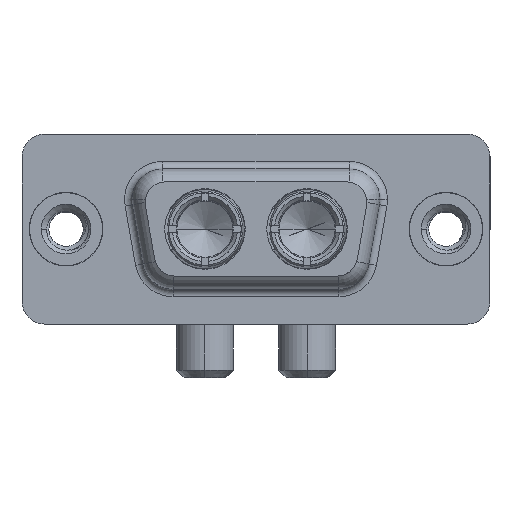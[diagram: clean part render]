
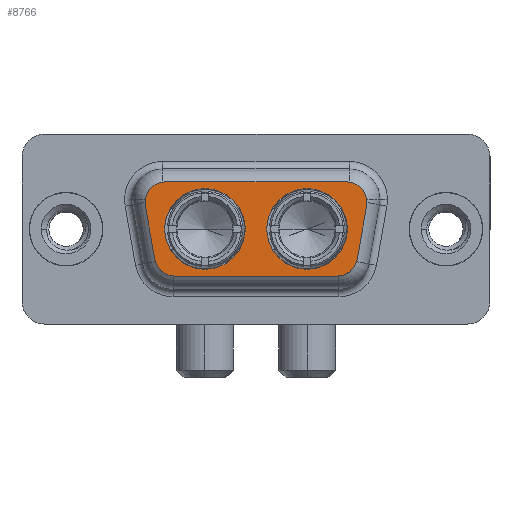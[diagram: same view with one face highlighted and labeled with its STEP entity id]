
A CAD part, top view. The second image highlights one B-rep face of the part: STEP entity #8766.
In plain terms, the highlighted planar face has unit normal (0, 0, 1).
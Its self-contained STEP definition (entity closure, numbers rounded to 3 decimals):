
#254 = DIRECTION ( 'NONE',  ( 0., 0., 1. ) ) ;
#322 = CARTESIAN_POINT ( 'NONE',  ( 9.14, 0., 6.2 ) ) ;
#446 = DIRECTION ( 'NONE',  ( 0., 0., 1. ) ) ;
#489 = VERTEX_POINT ( 'NONE', #9504 ) ;
#730 = CARTESIAN_POINT ( 'NONE',  ( 5.838, -1.984, 6.2 ) ) ;
#766 = CIRCLE ( 'NONE', #4537, 1.35 ) ;
#789 = VECTOR ( 'NONE', #3097, 1000. ) ;
#809 = CIRCLE ( 'NONE', #1787, 1.35 ) ;
#872 = ORIENTED_EDGE ( 'NONE', *, *, #11768, .T. ) ;
#908 = CARTESIAN_POINT ( 'NONE',  ( 7.167, -3.1, 6.2 ) ) ;
#1178 = EDGE_CURVE ( 'NONE', #6033, #6200, #5477, .T. ) ;
#1204 = VERTEX_POINT ( 'NONE', #908 ) ;
#1561 = DIRECTION ( 'NONE',  ( 0., 0., 1. ) ) ;
#1771 = VERTEX_POINT ( 'NONE', #10415 ) ;
#1781 = FACE_OUTER_BOUND ( 'NONE', #9798, .T. ) ;
#1787 = AXIS2_PLACEMENT_3D ( 'NONE', #3826, #3649, #8515 ) ;
#1828 = DIRECTION ( 'NONE',  ( 0., 0., 1. ) ) ;
#1871 = CARTESIAN_POINT ( 'NONE',  ( 18.45, 3.1, 6.2 ) ) ;
#1971 = AXIS2_PLACEMENT_3D ( 'NONE', #7436, #4839, #5643 ) ;
#2086 = DIRECTION ( 'NONE',  ( 0., 0., 1. ) ) ;
#2206 = DIRECTION ( 'NONE',  ( 1., 0., 0. ) ) ;
#2219 = LINE ( 'NONE', #11660, #789 ) ;
#2301 = ORIENTED_EDGE ( 'NONE', *, *, #11917, .T. ) ;
#2313 = ORIENTED_EDGE ( 'NONE', *, *, #7352, .T. ) ;
#2475 = EDGE_CURVE ( 'NONE', #4671, #489, #4843, .T. ) ;
#2494 = DIRECTION ( 'NONE',  ( 1., 0., 0. ) ) ;
#2518 = DIRECTION ( 'NONE',  ( 1., 0., 0. ) ) ;
#2545 = AXIS2_PLACEMENT_3D ( 'NONE', #7964, #2086, #4894 ) ;
#2638 = VERTEX_POINT ( 'NONE', #11983 ) ;
#2648 = AXIS2_PLACEMENT_3D ( 'NONE', #6838, #254, #4727 ) ;
#2899 = ORIENTED_EDGE ( 'NONE', *, *, #11365, .F. ) ;
#3053 = VERTEX_POINT ( 'NONE', #4282 ) ;
#3097 = DIRECTION ( 'NONE',  ( -1., 0., 0. ) ) ;
#3649 = DIRECTION ( 'NONE',  ( 0., 0., 1. ) ) ;
#3727 = CARTESIAN_POINT ( 'NONE',  ( 5.838, -1.984, 6.2 ) ) ;
#3826 = CARTESIAN_POINT ( 'NONE',  ( 17.833, -1.75, 6.2 ) ) ;
#3997 = VECTOR ( 'NONE', #9225, 1000. ) ;
#4095 = CARTESIAN_POINT ( 'NONE',  ( 18.51, 0., 6.2 ) ) ;
#4229 = DIRECTION ( 'NONE',  ( 1., 0., 0. ) ) ;
#4282 = CARTESIAN_POINT ( 'NONE',  ( 5.2, 1.75, 6.2 ) ) ;
#4336 = CIRCLE ( 'NONE', #6702, 1.35 ) ;
#4537 = AXIS2_PLACEMENT_3D ( 'NONE', #5172, #8915, #11566 ) ;
#4592 = FACE_BOUND ( 'NONE', #5334, .T. ) ;
#4664 = ORIENTED_EDGE ( 'NONE', *, *, #5208, .F. ) ;
#4671 = VERTEX_POINT ( 'NONE', #4095 ) ;
#4727 = DIRECTION ( 'NONE',  ( -1., 0., 0. ) ) ;
#4737 = CARTESIAN_POINT ( 'NONE',  ( 19.162, -1.984, 6.2 ) ) ;
#4807 = AXIS2_PLACEMENT_3D ( 'NONE', #9690, #6735, #2206 ) ;
#4839 = DIRECTION ( 'NONE',  ( 0., 0., -1. ) ) ;
#4843 = CIRCLE ( 'NONE', #7928, 2.65 ) ;
#4864 = CARTESIAN_POINT ( 'NONE',  ( 19.779, 1.516, 6.2 ) ) ;
#4894 = DIRECTION ( 'NONE',  ( 1., 0., 0. ) ) ;
#5019 = AXIS2_PLACEMENT_3D ( 'NONE', #322, #10841, #2494 ) ;
#5028 = VECTOR ( 'NONE', #5588, 1000. ) ;
#5172 = CARTESIAN_POINT ( 'NONE',  ( 18.45, 1.75, 6.2 ) ) ;
#5175 = CARTESIAN_POINT ( 'NONE',  ( 15.86, 0., 6.2 ) ) ;
#5208 = EDGE_CURVE ( 'NONE', #489, #4671, #6705, .T. ) ;
#5226 = LINE ( 'NONE', #10647, #9545 ) ;
#5334 = EDGE_LOOP ( 'NONE', ( #2899, #11483 ) ) ;
#5366 = DIRECTION ( 'NONE',  ( 1., 0., 0. ) ) ;
#5477 = LINE ( 'NONE', #12050, #3997 ) ;
#5588 = DIRECTION ( 'NONE',  ( 0.174, -0.985, 0. ) ) ;
#5643 = DIRECTION ( 'NONE',  ( -1., 0., 0. ) ) ;
#5976 = CARTESIAN_POINT ( 'NONE',  ( 6.55, 3.1, 6.2 ) ) ;
#6033 = VERTEX_POINT ( 'NONE', #4737 ) ;
#6120 = AXIS2_PLACEMENT_3D ( 'NONE', #10044, #1561, #5366 ) ;
#6200 = VERTEX_POINT ( 'NONE', #4864 ) ;
#6386 = CIRCLE ( 'NONE', #4807, 2.65 ) ;
#6391 = VERTEX_POINT ( 'NONE', #11848 ) ;
#6583 = VERTEX_POINT ( 'NONE', #11179 ) ;
#6657 = ORIENTED_EDGE ( 'NONE', *, *, #2475, .F. ) ;
#6702 = AXIS2_PLACEMENT_3D ( 'NONE', #8390, #1828, #2518 ) ;
#6705 = CIRCLE ( 'NONE', #2545, 2.65 ) ;
#6735 = DIRECTION ( 'NONE',  ( 0., 0., 1. ) ) ;
#6838 = CARTESIAN_POINT ( 'NONE',  ( 7.167, -1.75, 6.2 ) ) ;
#6967 = EDGE_CURVE ( 'NONE', #7615, #3053, #4336, .T. ) ;
#7352 = EDGE_CURVE ( 'NONE', #3053, #6583, #11415, .T. ) ;
#7436 = CARTESIAN_POINT ( 'NONE',  ( 7.167, -1.75, 6.2 ) ) ;
#7515 = VERTEX_POINT ( 'NONE', #1871 ) ;
#7576 = CIRCLE ( 'NONE', #5019, 2.65 ) ;
#7615 = VERTEX_POINT ( 'NONE', #5976 ) ;
#7689 = ORIENTED_EDGE ( 'NONE', *, *, #9335, .T. ) ;
#7714 = EDGE_CURVE ( 'NONE', #6200, #7515, #766, .T. ) ;
#7779 = CIRCLE ( 'NONE', #2648, 1.35 ) ;
#7883 = VERTEX_POINT ( 'NONE', #3727 ) ;
#7928 = AXIS2_PLACEMENT_3D ( 'NONE', #5175, #446, #7994 ) ;
#7964 = CARTESIAN_POINT ( 'NONE',  ( 15.86, 0., 6.2 ) ) ;
#7994 = DIRECTION ( 'NONE',  ( 1., 0., 0. ) ) ;
#8120 = ORIENTED_EDGE ( 'NONE', *, *, #8946, .T. ) ;
#8390 = CARTESIAN_POINT ( 'NONE',  ( 6.55, 1.75, 6.2 ) ) ;
#8515 = DIRECTION ( 'NONE',  ( -1., 0., 0. ) ) ;
#8766 = ADVANCED_FACE ( 'NONE', ( #9505, #4592, #1781 ), #9332, .F. ) ;
#8915 = DIRECTION ( 'NONE',  ( 0., 0., 1. ) ) ;
#8917 = EDGE_LOOP ( 'NONE', ( #6657, #4664 ) ) ;
#8946 = EDGE_CURVE ( 'NONE', #7515, #7615, #2219, .T. ) ;
#9206 = LINE ( 'NONE', #730, #5028 ) ;
#9225 = DIRECTION ( 'NONE',  ( 0.174, 0.985, 0. ) ) ;
#9233 = ORIENTED_EDGE ( 'NONE', *, *, #12069, .T. ) ;
#9332 = PLANE ( 'NONE',  #1971 ) ;
#9335 = EDGE_CURVE ( 'NONE', #2638, #6033, #809, .T. ) ;
#9504 = CARTESIAN_POINT ( 'NONE',  ( 13.21, 0., 6.2 ) ) ;
#9505 = FACE_BOUND ( 'NONE', #8917, .T. ) ;
#9545 = VECTOR ( 'NONE', #4229, 1000. ) ;
#9690 = CARTESIAN_POINT ( 'NONE',  ( 9.14, 0., 6.2 ) ) ;
#9798 = EDGE_LOOP ( 'NONE', ( #872, #2301, #7689, #11582, #11043, #8120, #10676, #2313, #9233 ) ) ;
#10044 = CARTESIAN_POINT ( 'NONE',  ( 6.55, 1.75, 6.2 ) ) ;
#10415 = CARTESIAN_POINT ( 'NONE',  ( 11.79, 0., 6.2 ) ) ;
#10647 = CARTESIAN_POINT ( 'NONE',  ( 17.833, -3.1, 6.2 ) ) ;
#10676 = ORIENTED_EDGE ( 'NONE', *, *, #6967, .T. ) ;
#10730 = EDGE_CURVE ( 'NONE', #6391, #1771, #6386, .T. ) ;
#10841 = DIRECTION ( 'NONE',  ( 0., 0., 1. ) ) ;
#11043 = ORIENTED_EDGE ( 'NONE', *, *, #7714, .T. ) ;
#11179 = CARTESIAN_POINT ( 'NONE',  ( 5.221, 1.516, 6.2 ) ) ;
#11365 = EDGE_CURVE ( 'NONE', #1771, #6391, #7576, .T. ) ;
#11415 = CIRCLE ( 'NONE', #6120, 1.35 ) ;
#11483 = ORIENTED_EDGE ( 'NONE', *, *, #10730, .F. ) ;
#11566 = DIRECTION ( 'NONE',  ( -1., 0., 0. ) ) ;
#11582 = ORIENTED_EDGE ( 'NONE', *, *, #1178, .T. ) ;
#11660 = CARTESIAN_POINT ( 'NONE',  ( 6.55, 3.1, 6.2 ) ) ;
#11768 = EDGE_CURVE ( 'NONE', #7883, #1204, #7779, .T. ) ;
#11848 = CARTESIAN_POINT ( 'NONE',  ( 6.49, 0., 6.2 ) ) ;
#11917 = EDGE_CURVE ( 'NONE', #1204, #2638, #5226, .T. ) ;
#11983 = CARTESIAN_POINT ( 'NONE',  ( 17.833, -3.1, 6.2 ) ) ;
#12050 = CARTESIAN_POINT ( 'NONE',  ( 19.779, 1.516, 6.2 ) ) ;
#12069 = EDGE_CURVE ( 'NONE', #6583, #7883, #9206, .T. ) ;
